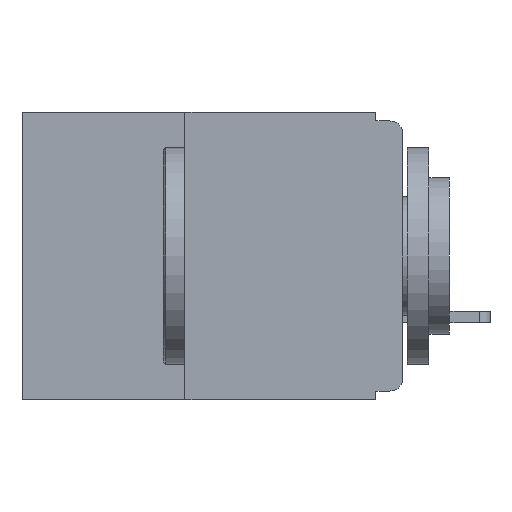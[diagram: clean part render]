
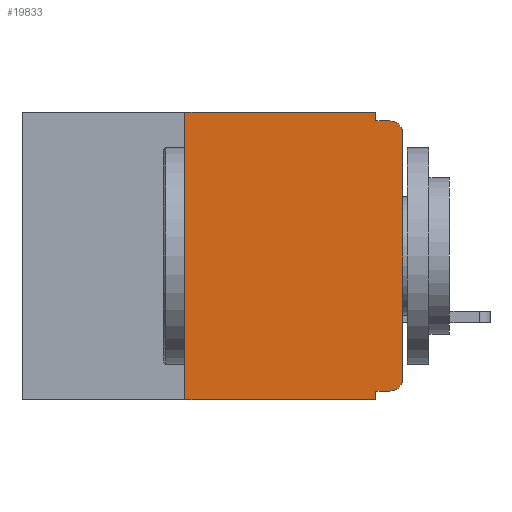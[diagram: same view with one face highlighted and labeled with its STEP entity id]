
A CAD part, left-side view. The second image highlights one B-rep face of the part: STEP entity #19833.
In plain terms, the highlighted planar face has unit normal (-1, 0, 0).
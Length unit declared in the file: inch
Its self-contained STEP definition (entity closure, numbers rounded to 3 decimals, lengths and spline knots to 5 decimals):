
#217 = EDGE_CURVE ( 'NONE', #20118, #28771, #21029, .T. ) ;
#819 = EDGE_CURVE ( 'NONE', #9805, #3851, #2943, .T. ) ;
#899 = AXIS2_PLACEMENT_3D ( 'NONE', #4010, #8207, #5381 ) ;
#1151 = DIRECTION ( 'NONE',  ( 0., 0., -1. ) ) ;
#2479 = CARTESIAN_POINT ( 'NONE',  ( 0., 0.031, -0.01 ) ) ;
#2943 = CIRCLE ( 'NONE', #899, 0.015 ) ;
#3486 = VERTEX_POINT ( 'NONE', #19125 ) ;
#3851 = VERTEX_POINT ( 'NONE', #13341 ) ;
#3897 = PLANE ( 'NONE',  #28456 ) ;
#4010 = CARTESIAN_POINT ( 'NONE',  ( 0., 0.015, -0.305 ) ) ;
#4385 = EDGE_CURVE ( 'NONE', #21400, #3486, #6483, .T. ) ;
#4435 = ORIENTED_EDGE ( 'NONE', *, *, #4385, .F. ) ;
#5381 = DIRECTION ( 'NONE',  ( 0., 0., -1. ) ) ;
#5421 = CARTESIAN_POINT ( 'NONE',  ( 0., 0., -0.01 ) ) ;
#5768 = VERTEX_POINT ( 'NONE', #20526 ) ;
#5822 = CARTESIAN_POINT ( 'NONE',  ( 0., 0.437, 0. ) ) ;
#5856 = DIRECTION ( 'NONE',  ( 0., -1., 0. ) ) ;
#6364 = DIRECTION ( 'NONE',  ( 0., 0., -1. ) ) ;
#6483 = LINE ( 'NONE', #5822, #25333 ) ;
#7500 = CARTESIAN_POINT ( 'NONE',  ( 0., 0., -0.32 ) ) ;
#7807 = EDGE_CURVE ( 'NONE', #12053, #5768, #10551, .T. ) ;
#8207 = DIRECTION ( 'NONE',  ( -1., 0., 0. ) ) ;
#8825 = CARTESIAN_POINT ( 'NONE',  ( 0., 0.015, -0.01 ) ) ;
#8862 = CARTESIAN_POINT ( 'NONE',  ( 0., 0.015, -0.025 ) ) ;
#9327 = CARTESIAN_POINT ( 'NONE',  ( 0., 0.031, -0.33 ) ) ;
#9446 = EDGE_CURVE ( 'NONE', #16648, #5768, #19014, .T. ) ;
#9494 = DIRECTION ( 'NONE',  ( 0., -1., 0. ) ) ;
#9805 = VERTEX_POINT ( 'NONE', #24443 ) ;
#10415 = LINE ( 'NONE', #24945, #23484 ) ;
#10551 = LINE ( 'NONE', #9327, #22082 ) ;
#11337 = DIRECTION ( 'NONE',  ( 0., 0., -1. ) ) ;
#11790 = DIRECTION ( 'NONE',  ( 0., 0., -1. ) ) ;
#12053 = VERTEX_POINT ( 'NONE', #12658 ) ;
#12359 = EDGE_CURVE ( 'NONE', #29333, #28771, #31391, .T. ) ;
#12475 = VECTOR ( 'NONE', #15781, 39.37008 ) ;
#12658 = CARTESIAN_POINT ( 'NONE',  ( 0., 0.031, -0.32 ) ) ;
#12753 = ORIENTED_EDGE ( 'NONE', *, *, #819, .T. ) ;
#13341 = CARTESIAN_POINT ( 'NONE',  ( 0., 0., -0.305 ) ) ;
#13407 = ORIENTED_EDGE ( 'NONE', *, *, #20982, .F. ) ;
#13530 = VECTOR ( 'NONE', #14923, 39.37008 ) ;
#14288 = CARTESIAN_POINT ( 'NONE',  ( 0., 0.25, -0.33 ) ) ;
#14923 = DIRECTION ( 'NONE',  ( 0., 1., 0. ) ) ;
#15781 = DIRECTION ( 'NONE',  ( 0., -1., 0. ) ) ;
#16046 = EDGE_CURVE ( 'NONE', #16648, #21400, #30181, .T. ) ;
#16099 = EDGE_LOOP ( 'NONE', ( #16260, #20733, #17872, #13407, #4435, #18239, #25267, #25010, #25349, #12753 ) ) ;
#16177 = CARTESIAN_POINT ( 'NONE',  ( 0., 0.437, 0. ) ) ;
#16260 = ORIENTED_EDGE ( 'NONE', *, *, #21622, .T. ) ;
#16648 = VERTEX_POINT ( 'NONE', #28834 ) ;
#16908 = LINE ( 'NONE', #30511, #22664 ) ;
#17565 = DIRECTION ( 'NONE',  ( 0., 0., 1. ) ) ;
#17872 = ORIENTED_EDGE ( 'NONE', *, *, #217, .F. ) ;
#17985 = VECTOR ( 'NONE', #28967, 39.37008 ) ;
#18239 = ORIENTED_EDGE ( 'NONE', *, *, #16046, .F. ) ;
#18961 = EDGE_CURVE ( 'NONE', #9805, #12053, #28107, .T. ) ;
#19014 = LINE ( 'NONE', #23082, #12475 ) ;
#19125 = CARTESIAN_POINT ( 'NONE',  ( 0., 0.031, 0. ) ) ;
#19176 = CARTESIAN_POINT ( 'NONE',  ( 0., 0.25, 0. ) ) ;
#19833 = ADVANCED_FACE ( 'NONE', ( #20017 ), #3897, .F. ) ;
#20017 = FACE_OUTER_BOUND ( 'NONE', #16099, .T. ) ;
#20118 = VERTEX_POINT ( 'NONE', #2479 ) ;
#20526 = CARTESIAN_POINT ( 'NONE',  ( 0., 0.031, -0.33 ) ) ;
#20733 = ORIENTED_EDGE ( 'NONE', *, *, #12359, .T. ) ;
#20982 = EDGE_CURVE ( 'NONE', #3486, #20118, #16908, .T. ) ;
#21029 = LINE ( 'NONE', #5421, #26768 ) ;
#21106 = DIRECTION ( 'NONE',  ( 1., 0., 0. ) ) ;
#21400 = VERTEX_POINT ( 'NONE', #19176 ) ;
#21622 = EDGE_CURVE ( 'NONE', #3851, #29333, #10415, .T. ) ;
#22082 = VECTOR ( 'NONE', #11790, 39.37008 ) ;
#22664 = VECTOR ( 'NONE', #1151, 39.37008 ) ;
#23082 = CARTESIAN_POINT ( 'NONE',  ( 0., 0.437, -0.33 ) ) ;
#23284 = CARTESIAN_POINT ( 'NONE',  ( 0., 0., -0.025 ) ) ;
#23484 = VECTOR ( 'NONE', #17565, 39.37008 ) ;
#24443 = CARTESIAN_POINT ( 'NONE',  ( 0., 0.015, -0.32 ) ) ;
#24945 = CARTESIAN_POINT ( 'NONE',  ( 0., 0., 0. ) ) ;
#25010 = ORIENTED_EDGE ( 'NONE', *, *, #7807, .F. ) ;
#25267 = ORIENTED_EDGE ( 'NONE', *, *, #9446, .T. ) ;
#25333 = VECTOR ( 'NONE', #5856, 39.37008 ) ;
#25349 = ORIENTED_EDGE ( 'NONE', *, *, #18961, .F. ) ;
#26058 = DIRECTION ( 'NONE',  ( -1., 0., 0. ) ) ;
#26768 = VECTOR ( 'NONE', #9494, 39.37008 ) ;
#26876 = AXIS2_PLACEMENT_3D ( 'NONE', #8862, #26058, #11337 ) ;
#28107 = LINE ( 'NONE', #7500, #13530 ) ;
#28456 = AXIS2_PLACEMENT_3D ( 'NONE', #16177, #21106, #6364 ) ;
#28771 = VERTEX_POINT ( 'NONE', #8825 ) ;
#28834 = CARTESIAN_POINT ( 'NONE',  ( 0., 0.25, -0.33 ) ) ;
#28967 = DIRECTION ( 'NONE',  ( 0., 0., 1. ) ) ;
#29333 = VERTEX_POINT ( 'NONE', #23284 ) ;
#30181 = LINE ( 'NONE', #14288, #17985 ) ;
#30511 = CARTESIAN_POINT ( 'NONE',  ( 0., 0.031, 0. ) ) ;
#31391 = CIRCLE ( 'NONE', #26876, 0.015 ) ;
